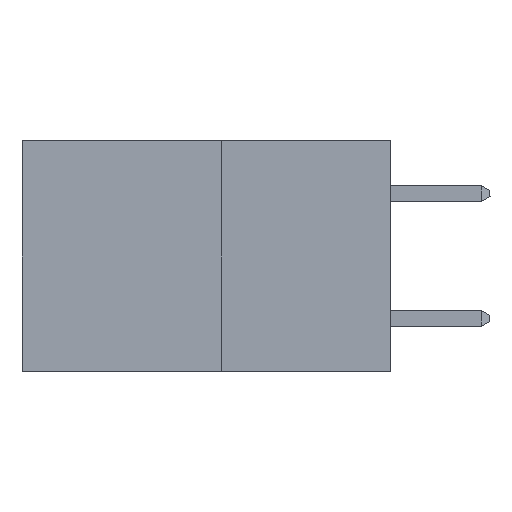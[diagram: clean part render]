
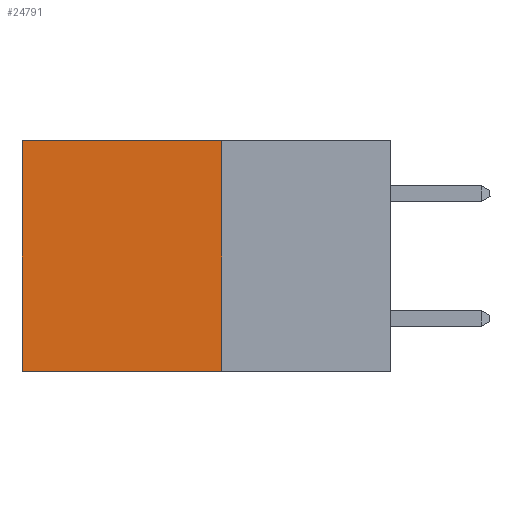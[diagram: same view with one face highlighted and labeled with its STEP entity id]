
A CAD part, left-side view. The second image highlights one B-rep face of the part: STEP entity #24791.
In plain terms, the highlighted planar face has unit normal (-1, 0, 0).
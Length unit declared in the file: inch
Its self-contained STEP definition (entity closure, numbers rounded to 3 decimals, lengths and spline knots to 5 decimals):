
#175 = CARTESIAN_POINT ( 'NONE',  ( 0.277, 0.27, -0.37 ) ) ;
#177 = CARTESIAN_POINT ( 'NONE',  ( 0.277, 0.27, 0. ) ) ;
#982 = CARTESIAN_POINT ( 'NONE',  ( 0.277, 0.27, -0.37 ) ) ;
#1446 = VERTEX_POINT ( 'NONE', #16345 ) ;
#1851 = AXIS2_PLACEMENT_3D ( 'NONE', #17993, #3385, #20449 ) ;
#2614 = VERTEX_POINT ( 'NONE', #982 ) ;
#2678 = DIRECTION ( 'NONE',  ( 0., 1., 0. ) ) ;
#3103 = ORIENTED_EDGE ( 'NONE', *, *, #16685, .T. ) ;
#3300 = VECTOR ( 'NONE', #20310, 39.37008 ) ;
#3385 = DIRECTION ( 'NONE',  ( 1., 0., 0. ) ) ;
#5724 = PLANE ( 'NONE',  #1851 ) ;
#5987 = VECTOR ( 'NONE', #8631, 39.37008 ) ;
#7080 = FACE_OUTER_BOUND ( 'NONE', #26746, .T. ) ;
#8631 = DIRECTION ( 'NONE',  ( 0., 0., -1. ) ) ;
#8670 = VECTOR ( 'NONE', #2678, 39.37008 ) ;
#8946 = ORIENTED_EDGE ( 'NONE', *, *, #13186, .T. ) ;
#9936 = DIRECTION ( 'NONE',  ( 0., 1., 0. ) ) ;
#10815 = LINE ( 'NONE', #26955, #23006 ) ;
#12476 = LINE ( 'NONE', #18355, #5987 ) ;
#13186 = EDGE_CURVE ( 'NONE', #27317, #1446, #10815, .T. ) ;
#14245 = ORIENTED_EDGE ( 'NONE', *, *, #23520, .F. ) ;
#14324 = CARTESIAN_POINT ( 'NONE',  ( 0.277, 0.59, -0.37 ) ) ;
#16345 = CARTESIAN_POINT ( 'NONE',  ( 0.277, 0.59, 0. ) ) ;
#16685 = EDGE_CURVE ( 'NONE', #1446, #27177, #22741, .T. ) ;
#17858 = CARTESIAN_POINT ( 'NONE',  ( 0.277, 0.59, -0.37 ) ) ;
#17993 = CARTESIAN_POINT ( 'NONE',  ( 0.277, 0.27, -0.37 ) ) ;
#18355 = CARTESIAN_POINT ( 'NONE',  ( 0.277, 0.27, -0.37 ) ) ;
#19000 = ORIENTED_EDGE ( 'NONE', *, *, #23204, .F. ) ;
#20310 = DIRECTION ( 'NONE',  ( 0., 0., -1. ) ) ;
#20449 = DIRECTION ( 'NONE',  ( 0., 0., -1. ) ) ;
#22741 = LINE ( 'NONE', #17858, #3300 ) ;
#23006 = VECTOR ( 'NONE', #9936, 39.37008 ) ;
#23204 = EDGE_CURVE ( 'NONE', #2614, #27177, #28839, .T. ) ;
#23520 = EDGE_CURVE ( 'NONE', #27317, #2614, #12476, .T. ) ;
#24791 = ADVANCED_FACE ( 'NONE', ( #7080 ), #5724, .F. ) ;
#26746 = EDGE_LOOP ( 'NONE', ( #3103, #19000, #14245, #8946 ) ) ;
#26955 = CARTESIAN_POINT ( 'NONE',  ( 0.277, 0.27, 0. ) ) ;
#27177 = VERTEX_POINT ( 'NONE', #14324 ) ;
#27317 = VERTEX_POINT ( 'NONE', #177 ) ;
#28839 = LINE ( 'NONE', #175, #8670 ) ;
